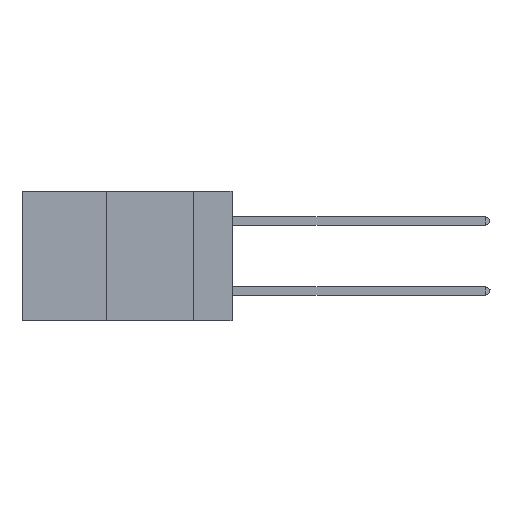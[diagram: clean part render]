
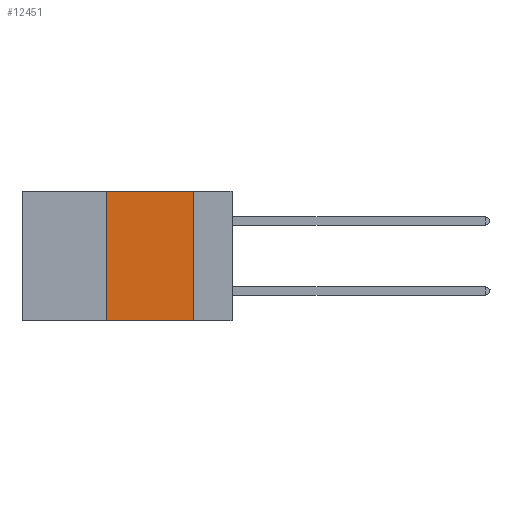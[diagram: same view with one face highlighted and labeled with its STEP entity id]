
A CAD part, left-side view. The second image highlights one B-rep face of the part: STEP entity #12451.
In plain terms, the highlighted planar face has unit normal (-1, 0, 0).
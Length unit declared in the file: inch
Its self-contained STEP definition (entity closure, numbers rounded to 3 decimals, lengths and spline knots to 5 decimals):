
#232 = CARTESIAN_POINT ( 'NONE',  ( 0., 0.11, -0.37 ) ) ;
#968 = DIRECTION ( 'NONE',  ( 1., 0., 0. ) ) ;
#1096 = EDGE_CURVE ( 'NONE', #13776, #1157, #9396, .T. ) ;
#1157 = VERTEX_POINT ( 'NONE', #15363 ) ;
#1803 = CARTESIAN_POINT ( 'NONE',  ( 0., 0.6, -0.37 ) ) ;
#2273 = ORIENTED_EDGE ( 'NONE', *, *, #11777, .F. ) ;
#2603 = LINE ( 'NONE', #1803, #5796 ) ;
#3597 = AXIS2_PLACEMENT_3D ( 'NONE', #9043, #968, #10352 ) ;
#4577 = VERTEX_POINT ( 'NONE', #232 ) ;
#5037 = PLANE ( 'NONE',  #3597 ) ;
#5490 = LINE ( 'NONE', #16226, #15298 ) ;
#5796 = VECTOR ( 'NONE', #12438, 39.37008 ) ;
#6855 = ORIENTED_EDGE ( 'NONE', *, *, #12408, .F. ) ;
#7187 = CARTESIAN_POINT ( 'NONE',  ( 0., 0.36, 0. ) ) ;
#7343 = DIRECTION ( 'NONE',  ( 0., 0., -1. ) ) ;
#9043 = CARTESIAN_POINT ( 'NONE',  ( 0., 0.6, 0. ) ) ;
#9396 = LINE ( 'NONE', #13046, #16055 ) ;
#9838 = ORIENTED_EDGE ( 'NONE', *, *, #1096, .F. ) ;
#10055 = EDGE_CURVE ( 'NONE', #10466, #4577, #2603, .T. ) ;
#10241 = DIRECTION ( 'NONE',  ( 0., -1., 0. ) ) ;
#10352 = DIRECTION ( 'NONE',  ( 0., 0., -1. ) ) ;
#10466 = VERTEX_POINT ( 'NONE', #16385 ) ;
#11267 = FACE_OUTER_BOUND ( 'NONE', #15237, .T. ) ;
#11354 = ORIENTED_EDGE ( 'NONE', *, *, #10055, .T. ) ;
#11777 = EDGE_CURVE ( 'NONE', #10466, #13776, #15922, .T. ) ;
#12408 = EDGE_CURVE ( 'NONE', #1157, #4577, #5490, .T. ) ;
#12438 = DIRECTION ( 'NONE',  ( 0., -1., 0. ) ) ;
#12451 = ADVANCED_FACE ( 'NONE', ( #11267 ), #5037, .F. ) ;
#12656 = DIRECTION ( 'NONE',  ( 0., 0., 1. ) ) ;
#13046 = CARTESIAN_POINT ( 'NONE',  ( 0., 0.6, 0. ) ) ;
#13776 = VERTEX_POINT ( 'NONE', #7187 ) ;
#15100 = CARTESIAN_POINT ( 'NONE',  ( 0., 0.36, 0. ) ) ;
#15237 = EDGE_LOOP ( 'NONE', ( #6855, #9838, #2273, #11354 ) ) ;
#15298 = VECTOR ( 'NONE', #7343, 39.37008 ) ;
#15363 = CARTESIAN_POINT ( 'NONE',  ( 0., 0.11, 0. ) ) ;
#15534 = VECTOR ( 'NONE', #12656, 39.37008 ) ;
#15922 = LINE ( 'NONE', #15100, #15534 ) ;
#16055 = VECTOR ( 'NONE', #10241, 39.37008 ) ;
#16226 = CARTESIAN_POINT ( 'NONE',  ( 0., 0.11, 0. ) ) ;
#16385 = CARTESIAN_POINT ( 'NONE',  ( 0., 0.36, -0.37 ) ) ;
